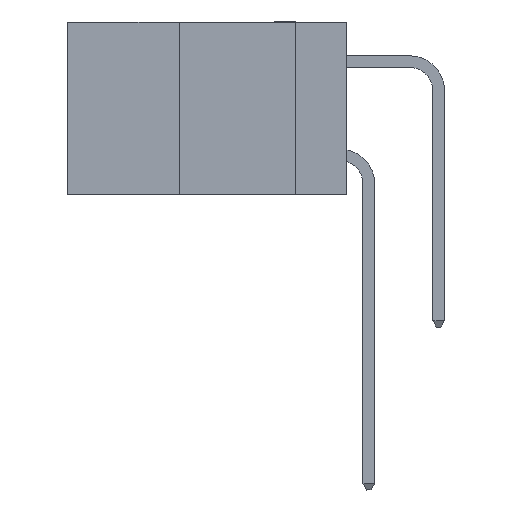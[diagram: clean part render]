
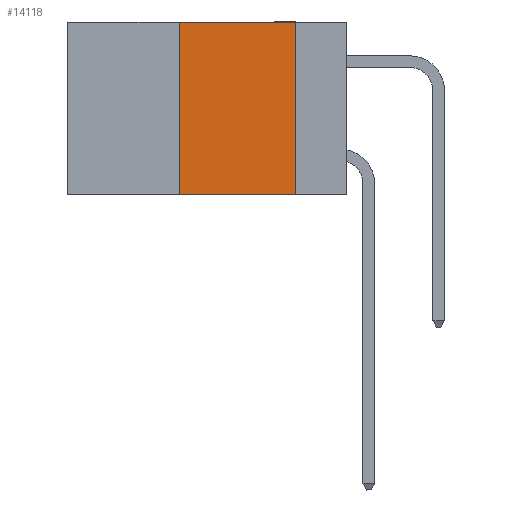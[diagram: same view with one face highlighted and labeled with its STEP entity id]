
A CAD part, left-side view. The second image highlights one B-rep face of the part: STEP entity #14118.
In plain terms, the highlighted planar face has unit normal (-1, 0, 0).
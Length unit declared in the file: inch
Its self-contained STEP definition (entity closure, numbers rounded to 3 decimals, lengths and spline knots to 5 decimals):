
#189 = CARTESIAN_POINT ( 'NONE',  ( 0., 0.6, -0.37 ) ) ;
#325 = VERTEX_POINT ( 'NONE', #9280 ) ;
#1191 = CARTESIAN_POINT ( 'NONE',  ( 0., 0.36, 0. ) ) ;
#2268 = VERTEX_POINT ( 'NONE', #3343 ) ;
#2553 = CARTESIAN_POINT ( 'NONE',  ( 0., 0.11, 0. ) ) ;
#2755 = LINE ( 'NONE', #2553, #14417 ) ;
#2881 = LINE ( 'NONE', #4662, #18072 ) ;
#3343 = CARTESIAN_POINT ( 'NONE',  ( 0., 0.36, -0.37 ) ) ;
#4098 = DIRECTION ( 'NONE',  ( 1., 0., 0. ) ) ;
#4662 = CARTESIAN_POINT ( 'NONE',  ( 0., 0.6, 0. ) ) ;
#6071 = DIRECTION ( 'NONE',  ( 0., -1., 0. ) ) ;
#6734 = VERTEX_POINT ( 'NONE', #9253 ) ;
#8663 = DIRECTION ( 'NONE',  ( 0., 0., -1. ) ) ;
#8702 = ORIENTED_EDGE ( 'NONE', *, *, #16954, .T. ) ;
#9253 = CARTESIAN_POINT ( 'NONE',  ( 0., 0.11, -0.37 ) ) ;
#9280 = CARTESIAN_POINT ( 'NONE',  ( 0., 0.36, 0. ) ) ;
#9882 = DIRECTION ( 'NONE',  ( 0., 0., -1. ) ) ;
#10017 = LINE ( 'NONE', #189, #16636 ) ;
#10829 = VERTEX_POINT ( 'NONE', #17682 ) ;
#10834 = ORIENTED_EDGE ( 'NONE', *, *, #12370, .F. ) ;
#12370 = EDGE_CURVE ( 'NONE', #2268, #325, #12448, .T. ) ;
#12448 = LINE ( 'NONE', #1191, #18453 ) ;
#12952 = CARTESIAN_POINT ( 'NONE',  ( 0., 0.6, 0. ) ) ;
#13084 = FACE_OUTER_BOUND ( 'NONE', #13988, .T. ) ;
#13204 = DIRECTION ( 'NONE',  ( 0., -1., 0. ) ) ;
#13988 = EDGE_LOOP ( 'NONE', ( #14762, #18272, #10834, #8702 ) ) ;
#14118 = ADVANCED_FACE ( 'NONE', ( #13084 ), #14591, .F. ) ;
#14417 = VECTOR ( 'NONE', #9882, 39.37008 ) ;
#14591 = PLANE ( 'NONE',  #16526 ) ;
#14650 = EDGE_CURVE ( 'NONE', #10829, #6734, #2755, .T. ) ;
#14762 = ORIENTED_EDGE ( 'NONE', *, *, #14650, .F. ) ;
#16526 = AXIS2_PLACEMENT_3D ( 'NONE', #12952, #4098, #8663 ) ;
#16636 = VECTOR ( 'NONE', #6071, 39.37008 ) ;
#16873 = EDGE_CURVE ( 'NONE', #325, #10829, #2881, .T. ) ;
#16954 = EDGE_CURVE ( 'NONE', #2268, #6734, #10017, .T. ) ;
#17202 = DIRECTION ( 'NONE',  ( 0., 0., 1. ) ) ;
#17682 = CARTESIAN_POINT ( 'NONE',  ( 0., 0.11, 0. ) ) ;
#18072 = VECTOR ( 'NONE', #13204, 39.37008 ) ;
#18272 = ORIENTED_EDGE ( 'NONE', *, *, #16873, .F. ) ;
#18453 = VECTOR ( 'NONE', #17202, 39.37008 ) ;
